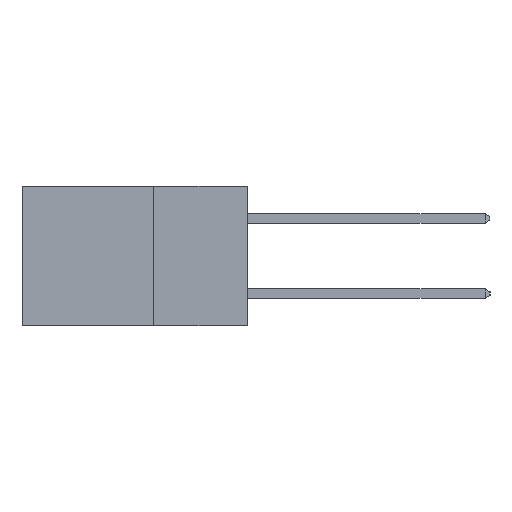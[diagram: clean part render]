
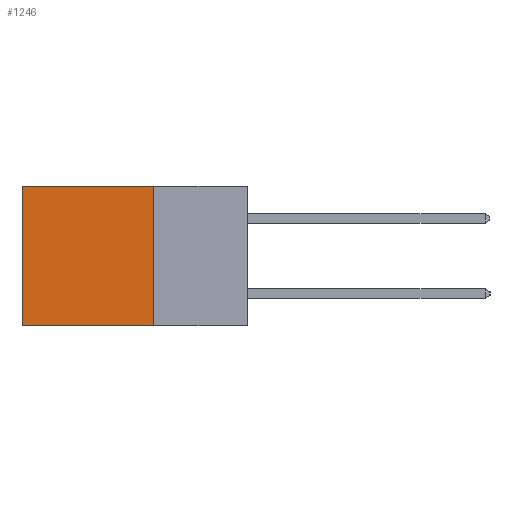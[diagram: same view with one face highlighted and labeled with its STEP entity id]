
A CAD part, left-side view. The second image highlights one B-rep face of the part: STEP entity #1246.
In plain terms, the highlighted planar face has unit normal (-1, 0, 0).
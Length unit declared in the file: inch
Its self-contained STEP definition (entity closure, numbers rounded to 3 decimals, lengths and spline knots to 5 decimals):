
#154 = VECTOR ( 'NONE', #10408, 39.37008 ) ;
#350 = LINE ( 'NONE', #6673, #4139 ) ;
#563 = FACE_OUTER_BOUND ( 'NONE', #8066, .T. ) ;
#619 = DIRECTION ( 'NONE',  ( 0., 0., -1. ) ) ;
#1246 = ADVANCED_FACE ( 'NONE', ( #563 ), #8177, .F. ) ;
#1412 = ORIENTED_EDGE ( 'NONE', *, *, #9877, .F. ) ;
#1422 = VERTEX_POINT ( 'NONE', #6845 ) ;
#2173 = EDGE_CURVE ( 'NONE', #4833, #4619, #6985, .T. ) ;
#2517 = EDGE_CURVE ( 'NONE', #1422, #2901, #5431, .T. ) ;
#2901 = VERTEX_POINT ( 'NONE', #3245 ) ;
#3187 = DIRECTION ( 'NONE',  ( 0., 0., -1. ) ) ;
#3245 = CARTESIAN_POINT ( 'NONE',  ( 0.2615, 0.6, 0. ) ) ;
#3419 = VECTOR ( 'NONE', #9817, 39.37008 ) ;
#3512 = ORIENTED_EDGE ( 'NONE', *, *, #2517, .T. ) ;
#4139 = VECTOR ( 'NONE', #3187, 39.37008 ) ;
#4619 = VERTEX_POINT ( 'NONE', #10050 ) ;
#4833 = VERTEX_POINT ( 'NONE', #6908 ) ;
#5431 = LINE ( 'NONE', #8483, #9406 ) ;
#5528 = ORIENTED_EDGE ( 'NONE', *, *, #2173, .F. ) ;
#5895 = AXIS2_PLACEMENT_3D ( 'NONE', #7996, #10495, #619 ) ;
#6673 = CARTESIAN_POINT ( 'NONE',  ( 0.2615, 0.25, -0.37 ) ) ;
#6845 = CARTESIAN_POINT ( 'NONE',  ( 0.2615, 0.25, 0. ) ) ;
#6908 = CARTESIAN_POINT ( 'NONE',  ( 0.2615, 0.25, -0.37 ) ) ;
#6985 = LINE ( 'NONE', #8298, #154 ) ;
#7928 = LINE ( 'NONE', #9057, #3419 ) ;
#7996 = CARTESIAN_POINT ( 'NONE',  ( 0.2615, 0.25, -0.37 ) ) ;
#8031 = DIRECTION ( 'NONE',  ( 0., 1., 0. ) ) ;
#8066 = EDGE_LOOP ( 'NONE', ( #8793, #5528, #1412, #3512 ) ) ;
#8177 = PLANE ( 'NONE',  #5895 ) ;
#8298 = CARTESIAN_POINT ( 'NONE',  ( 0.2615, 0.25, -0.37 ) ) ;
#8483 = CARTESIAN_POINT ( 'NONE',  ( 0.2615, 0.25, 0. ) ) ;
#8793 = ORIENTED_EDGE ( 'NONE', *, *, #9277, .T. ) ;
#9057 = CARTESIAN_POINT ( 'NONE',  ( 0.2615, 0.6, -0.37 ) ) ;
#9277 = EDGE_CURVE ( 'NONE', #2901, #4619, #7928, .T. ) ;
#9406 = VECTOR ( 'NONE', #8031, 39.37008 ) ;
#9817 = DIRECTION ( 'NONE',  ( 0., 0., -1. ) ) ;
#9877 = EDGE_CURVE ( 'NONE', #1422, #4833, #350, .T. ) ;
#10050 = CARTESIAN_POINT ( 'NONE',  ( 0.2615, 0.6, -0.37 ) ) ;
#10408 = DIRECTION ( 'NONE',  ( 0., 1., 0. ) ) ;
#10495 = DIRECTION ( 'NONE',  ( 1., 0., 0. ) ) ;
